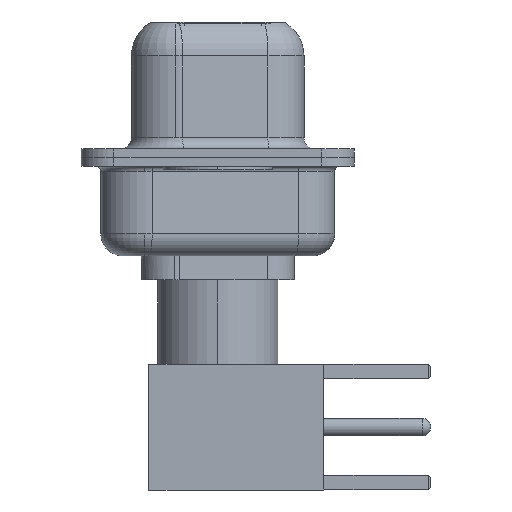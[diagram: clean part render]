
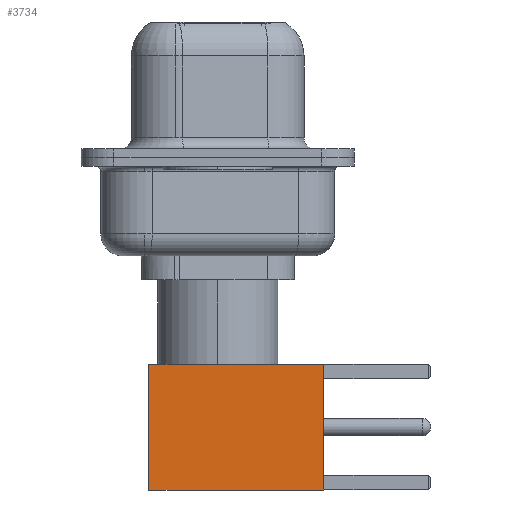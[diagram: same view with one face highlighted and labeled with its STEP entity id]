
A CAD part, left-side view. The second image highlights one B-rep face of the part: STEP entity #3734.
In plain terms, the highlighted face is planar.
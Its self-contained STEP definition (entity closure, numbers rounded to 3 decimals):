
#166 = EDGE_CURVE ( 'NONE', #7445, #11049, #2985, .T. ) ;
#450 = CARTESIAN_POINT ( 'NONE',  ( 0., 2.875, 8. ) ) ;
#614 = EDGE_CURVE ( 'NONE', #672, #11049, #7228, .T. ) ;
#616 = PLANE ( 'NONE',  #7942 ) ;
#672 = VERTEX_POINT ( 'NONE', #13713 ) ;
#1336 = VERTEX_POINT ( 'NONE', #13369 ) ;
#1611 = CARTESIAN_POINT ( 'NONE',  ( 2.875, 2.875, 0. ) ) ;
#2856 = FACE_OUTER_BOUND ( 'NONE', #6905, .T. ) ;
#2904 = DIRECTION ( 'NONE',  ( 0., 0., -1. ) ) ;
#2924 = CARTESIAN_POINT ( 'NONE',  ( 2.875, 2.875, 0. ) ) ;
#2985 = LINE ( 'NONE', #3918, #3499 ) ;
#3499 = VECTOR ( 'NONE', #10678, 1000. ) ;
#3734 = ADVANCED_FACE ( 'NONE', ( #2856 ), #616, .T. ) ;
#3918 = CARTESIAN_POINT ( 'NONE',  ( 0., 2.875, 0. ) ) ;
#4879 = DIRECTION ( 'NONE',  ( 0., 0., 1. ) ) ;
#5167 = VECTOR ( 'NONE', #12773, 1000. ) ;
#5363 = DIRECTION ( 'NONE',  ( 0., 0., -1. ) ) ;
#5707 = ORIENTED_EDGE ( 'NONE', *, *, #614, .F. ) ;
#5998 = ORIENTED_EDGE ( 'NONE', *, *, #166, .T. ) ;
#6905 = EDGE_LOOP ( 'NONE', ( #9771, #5998, #5707, #9245 ) ) ;
#7228 = LINE ( 'NONE', #12840, #14076 ) ;
#7445 = VERTEX_POINT ( 'NONE', #1611 ) ;
#7942 = AXIS2_PLACEMENT_3D ( 'NONE', #2924, #11759, #4879 ) ;
#9145 = EDGE_CURVE ( 'NONE', #1336, #7445, #14213, .T. ) ;
#9245 = ORIENTED_EDGE ( 'NONE', *, *, #9530, .F. ) ;
#9357 = CARTESIAN_POINT ( 'NONE',  ( -2.875, 2.875, 0. ) ) ;
#9530 = EDGE_CURVE ( 'NONE', #1336, #672, #10524, .T. ) ;
#9771 = ORIENTED_EDGE ( 'NONE', *, *, #9145, .T. ) ;
#10524 = LINE ( 'NONE', #450, #5167 ) ;
#10678 = DIRECTION ( 'NONE',  ( -1., 0., 0. ) ) ;
#10747 = CARTESIAN_POINT ( 'NONE',  ( 2.875, 2.875, 0. ) ) ;
#11049 = VERTEX_POINT ( 'NONE', #9357 ) ;
#11759 = DIRECTION ( 'NONE',  ( 0., 1., 0. ) ) ;
#12021 = VECTOR ( 'NONE', #5363, 1000. ) ;
#12773 = DIRECTION ( 'NONE',  ( -1., 0., 0. ) ) ;
#12840 = CARTESIAN_POINT ( 'NONE',  ( -2.875, 2.875, 0. ) ) ;
#13369 = CARTESIAN_POINT ( 'NONE',  ( 2.875, 2.875, 8. ) ) ;
#13713 = CARTESIAN_POINT ( 'NONE',  ( -2.875, 2.875, 8. ) ) ;
#14076 = VECTOR ( 'NONE', #2904, 1000. ) ;
#14213 = LINE ( 'NONE', #10747, #12021 ) ;
